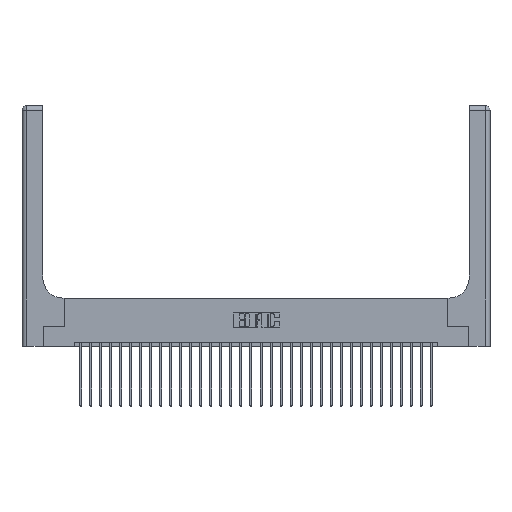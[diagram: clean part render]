
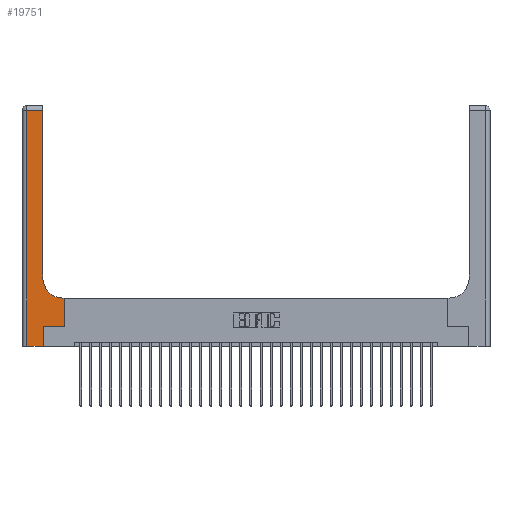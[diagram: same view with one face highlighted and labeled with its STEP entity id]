
A CAD part, top view. The second image highlights one B-rep face of the part: STEP entity #19751.
In plain terms, the highlighted planar face has unit normal (0, 0, 1).
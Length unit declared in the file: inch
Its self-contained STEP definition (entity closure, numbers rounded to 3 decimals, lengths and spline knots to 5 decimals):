
#195 = VECTOR ( 'NONE', #2462, 39.37008 ) ;
#292 = EDGE_CURVE ( 'NONE', #22188, #797, #24545, .T. ) ;
#716 = EDGE_CURVE ( 'NONE', #11319, #26152, #21979, .T. ) ;
#797 = VERTEX_POINT ( 'NONE', #29656 ) ;
#1752 = CARTESIAN_POINT ( 'NONE',  ( 0.51, 0.85, 0.37 ) ) ;
#1763 = ORIENTED_EDGE ( 'NONE', *, *, #28488, .T. ) ;
#1943 = CARTESIAN_POINT ( 'NONE',  ( 0.26, 3., 0.37 ) ) ;
#2462 = DIRECTION ( 'NONE',  ( 0., 1., 0. ) ) ;
#2853 = EDGE_CURVE ( 'NONE', #23201, #22188, #18402, .T. ) ;
#3312 = CARTESIAN_POINT ( 'NONE',  ( 0.26, 0.6, 0.37 ) ) ;
#3438 = ORIENTED_EDGE ( 'NONE', *, *, #22029, .T. ) ;
#3780 = EDGE_CURVE ( 'NONE', #26152, #21643, #29853, .T. ) ;
#4203 = VERTEX_POINT ( 'NONE', #21947 ) ;
#4960 = CARTESIAN_POINT ( 'NONE',  ( 0., 3., 0.37 ) ) ;
#5472 = CARTESIAN_POINT ( 'NONE',  ( 0., 2.94, 0.37 ) ) ;
#5568 = EDGE_CURVE ( 'NONE', #4203, #19443, #21461, .T. ) ;
#6651 = ORIENTED_EDGE ( 'NONE', *, *, #23533, .T. ) ;
#7416 = CARTESIAN_POINT ( 'NONE',  ( 0.265, 0.25, 0.37 ) ) ;
#7654 = ORIENTED_EDGE ( 'NONE', *, *, #716, .T. ) ;
#7655 = VECTOR ( 'NONE', #28628, 39.37008 ) ;
#7751 = VECTOR ( 'NONE', #25146, 39.37008 ) ;
#7841 = CARTESIAN_POINT ( 'NONE',  ( 0.51, 0.6, 0.37 ) ) ;
#7848 = FACE_OUTER_BOUND ( 'NONE', #8409, .T. ) ;
#7905 = LINE ( 'NONE', #5472, #26025 ) ;
#8409 = EDGE_LOOP ( 'NONE', ( #28899, #1763, #12055, #3438, #11430, #11068, #28390, #6651, #7654 ) ) ;
#8816 = CARTESIAN_POINT ( 'NONE',  ( 0., 0., 0.37 ) ) ;
#9396 = AXIS2_PLACEMENT_3D ( 'NONE', #1752, #29352, #22675 ) ;
#9588 = DIRECTION ( 'NONE',  ( -1., 0., 0. ) ) ;
#10288 = VECTOR ( 'NONE', #22867, 39.37008 ) ;
#11068 = ORIENTED_EDGE ( 'NONE', *, *, #292, .T. ) ;
#11319 = VERTEX_POINT ( 'NONE', #7841 ) ;
#11430 = ORIENTED_EDGE ( 'NONE', *, *, #2853, .T. ) ;
#11745 = CARTESIAN_POINT ( 'NONE',  ( 0.265, 0., 0.37 ) ) ;
#12055 = ORIENTED_EDGE ( 'NONE', *, *, #5568, .T. ) ;
#12233 = DIRECTION ( 'NONE',  ( 0., -1., 0. ) ) ;
#12546 = DIRECTION ( 'NONE',  ( -1., 0., 0. ) ) ;
#13674 = DIRECTION ( 'NONE',  ( 0., 1., 0. ) ) ;
#14086 = CARTESIAN_POINT ( 'NONE',  ( 0.528, 0.6, 0.37 ) ) ;
#14215 = DIRECTION ( 'NONE',  ( 0., 0., -1. ) ) ;
#15149 = EDGE_CURVE ( 'NONE', #797, #27012, #20481, .T. ) ;
#15906 = CARTESIAN_POINT ( 'NONE',  ( 0.265, 0.25, 0.37 ) ) ;
#16379 = LINE ( 'NONE', #8816, #25477 ) ;
#16611 = VECTOR ( 'NONE', #13674, 39.37008 ) ;
#16617 = CARTESIAN_POINT ( 'NONE',  ( 0.26, 2.94, 0.37 ) ) ;
#18402 = LINE ( 'NONE', #11745, #195 ) ;
#19359 = PLANE ( 'NONE',  #22501 ) ;
#19425 = CARTESIAN_POINT ( 'NONE',  ( 0.265, 0., 0.37 ) ) ;
#19443 = VERTEX_POINT ( 'NONE', #27116 ) ;
#19751 = ADVANCED_FACE ( 'NONE', ( #7848 ), #19359, .F. ) ;
#20481 = LINE ( 'NONE', #25177, #16611 ) ;
#20959 = CARTESIAN_POINT ( 'NONE',  ( 0.26, 0.85, 0.37 ) ) ;
#21461 = LINE ( 'NONE', #26319, #28312 ) ;
#21643 = VERTEX_POINT ( 'NONE', #16617 ) ;
#21947 = CARTESIAN_POINT ( 'NONE',  ( 0.06, 2.94, 0.37 ) ) ;
#21979 = CIRCLE ( 'NONE', #9396, 0.25 ) ;
#22029 = EDGE_CURVE ( 'NONE', #19443, #23201, #16379, .T. ) ;
#22188 = VERTEX_POINT ( 'NONE', #7416 ) ;
#22501 = AXIS2_PLACEMENT_3D ( 'NONE', #4960, #14215, #12546 ) ;
#22675 = DIRECTION ( 'NONE',  ( 1., 0., 0. ) ) ;
#22867 = DIRECTION ( 'NONE',  ( 0., 1., 0. ) ) ;
#23201 = VERTEX_POINT ( 'NONE', #19425 ) ;
#23533 = EDGE_CURVE ( 'NONE', #27012, #11319, #25909, .T. ) ;
#24545 = LINE ( 'NONE', #15906, #7751 ) ;
#25146 = DIRECTION ( 'NONE',  ( 1., 0., 0. ) ) ;
#25177 = CARTESIAN_POINT ( 'NONE',  ( 0.528, 0.25, 0.37 ) ) ;
#25477 = VECTOR ( 'NONE', #25609, 39.37008 ) ;
#25609 = DIRECTION ( 'NONE',  ( 1., 0., 0. ) ) ;
#25909 = LINE ( 'NONE', #3312, #7655 ) ;
#26025 = VECTOR ( 'NONE', #9588, 39.37008 ) ;
#26152 = VERTEX_POINT ( 'NONE', #20959 ) ;
#26319 = CARTESIAN_POINT ( 'NONE',  ( 0.06, 3., 0.37 ) ) ;
#27012 = VERTEX_POINT ( 'NONE', #14086 ) ;
#27116 = CARTESIAN_POINT ( 'NONE',  ( 0.06, 0., 0.37 ) ) ;
#28312 = VECTOR ( 'NONE', #12233, 39.37008 ) ;
#28390 = ORIENTED_EDGE ( 'NONE', *, *, #15149, .T. ) ;
#28488 = EDGE_CURVE ( 'NONE', #21643, #4203, #7905, .T. ) ;
#28628 = DIRECTION ( 'NONE',  ( -1., 0., 0. ) ) ;
#28899 = ORIENTED_EDGE ( 'NONE', *, *, #3780, .T. ) ;
#29352 = DIRECTION ( 'NONE',  ( 0., 0., -1. ) ) ;
#29656 = CARTESIAN_POINT ( 'NONE',  ( 0.528, 0.25, 0.37 ) ) ;
#29853 = LINE ( 'NONE', #1943, #10288 ) ;
